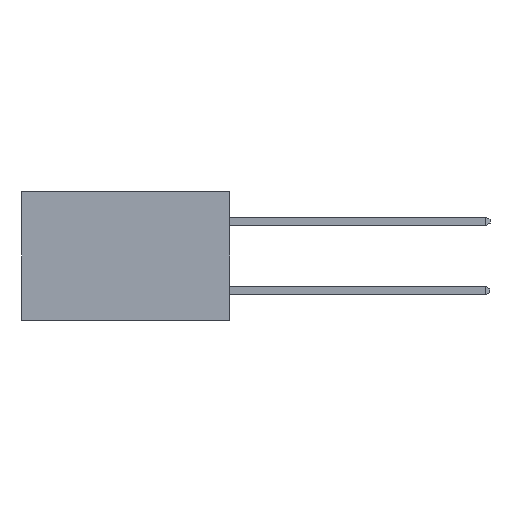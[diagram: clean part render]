
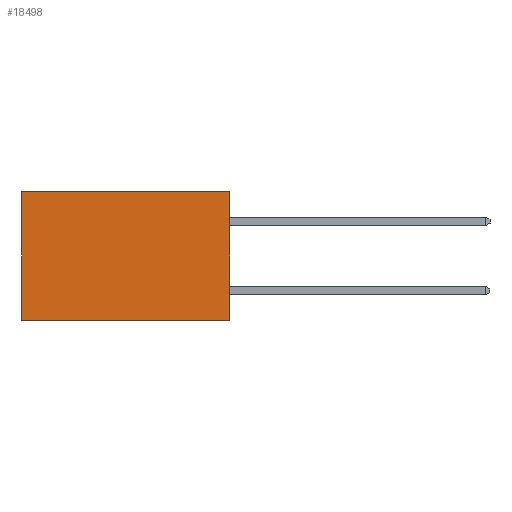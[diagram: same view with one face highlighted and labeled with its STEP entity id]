
A CAD part, left-side view. The second image highlights one B-rep face of the part: STEP entity #18498.
In plain terms, the highlighted planar face has unit normal (-1, 0, 0).
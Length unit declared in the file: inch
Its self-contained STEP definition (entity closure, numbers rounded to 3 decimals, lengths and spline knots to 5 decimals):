
#253 = CARTESIAN_POINT ( 'NONE',  ( 0.298, 0., 0. ) ) ;
#1426 = CARTESIAN_POINT ( 'NONE',  ( 0.298, 0., 0. ) ) ;
#1556 = PLANE ( 'NONE',  #8945 ) ;
#1568 = CARTESIAN_POINT ( 'NONE',  ( 0.298, 0.6, 0. ) ) ;
#1575 = CARTESIAN_POINT ( 'NONE',  ( 0.298, 0., -0.37 ) ) ;
#2630 = CARTESIAN_POINT ( 'NONE',  ( 0.298, 0., 0. ) ) ;
#3134 = ORIENTED_EDGE ( 'NONE', *, *, #11621, .F. ) ;
#3983 = FACE_OUTER_BOUND ( 'NONE', #7855, .T. ) ;
#4837 = CARTESIAN_POINT ( 'NONE',  ( 0.298, 0., -0.37 ) ) ;
#5076 = DIRECTION ( 'NONE',  ( 0., 0., -1. ) ) ;
#5237 = DIRECTION ( 'NONE',  ( 1., 0., 0. ) ) ;
#5531 = VECTOR ( 'NONE', #5076, 39.37008 ) ;
#6253 = CARTESIAN_POINT ( 'NONE',  ( 0.298, 0.6, -0.37 ) ) ;
#6757 = VERTEX_POINT ( 'NONE', #1568 ) ;
#6999 = LINE ( 'NONE', #4837, #20323 ) ;
#7852 = VECTOR ( 'NONE', #11944, 39.37008 ) ;
#7855 = EDGE_LOOP ( 'NONE', ( #11412, #13871, #3134, #12021 ) ) ;
#7926 = DIRECTION ( 'NONE',  ( 0., 0., -1. ) ) ;
#8945 = AXIS2_PLACEMENT_3D ( 'NONE', #15700, #5237, #17419 ) ;
#9038 = LINE ( 'NONE', #15537, #5531 ) ;
#9206 = VECTOR ( 'NONE', #7926, 39.37008 ) ;
#11385 = VERTEX_POINT ( 'NONE', #253 ) ;
#11412 = ORIENTED_EDGE ( 'NONE', *, *, #14976, .T. ) ;
#11621 = EDGE_CURVE ( 'NONE', #11385, #19896, #13869, .T. ) ;
#11944 = DIRECTION ( 'NONE',  ( 0., 1., 0. ) ) ;
#12021 = ORIENTED_EDGE ( 'NONE', *, *, #17902, .T. ) ;
#13011 = LINE ( 'NONE', #1426, #7852 ) ;
#13503 = DIRECTION ( 'NONE',  ( 0., 1., 0. ) ) ;
#13869 = LINE ( 'NONE', #2630, #9206 ) ;
#13871 = ORIENTED_EDGE ( 'NONE', *, *, #19048, .F. ) ;
#14763 = VERTEX_POINT ( 'NONE', #6253 ) ;
#14976 = EDGE_CURVE ( 'NONE', #6757, #14763, #9038, .T. ) ;
#15537 = CARTESIAN_POINT ( 'NONE',  ( 0.298, 0.6, 0. ) ) ;
#15700 = CARTESIAN_POINT ( 'NONE',  ( 0.298, 0., 0. ) ) ;
#17419 = DIRECTION ( 'NONE',  ( 0., 0., -1. ) ) ;
#17902 = EDGE_CURVE ( 'NONE', #11385, #6757, #13011, .T. ) ;
#18498 = ADVANCED_FACE ( 'NONE', ( #3983 ), #1556, .F. ) ;
#19048 = EDGE_CURVE ( 'NONE', #19896, #14763, #6999, .T. ) ;
#19896 = VERTEX_POINT ( 'NONE', #1575 ) ;
#20323 = VECTOR ( 'NONE', #13503, 39.37008 ) ;
